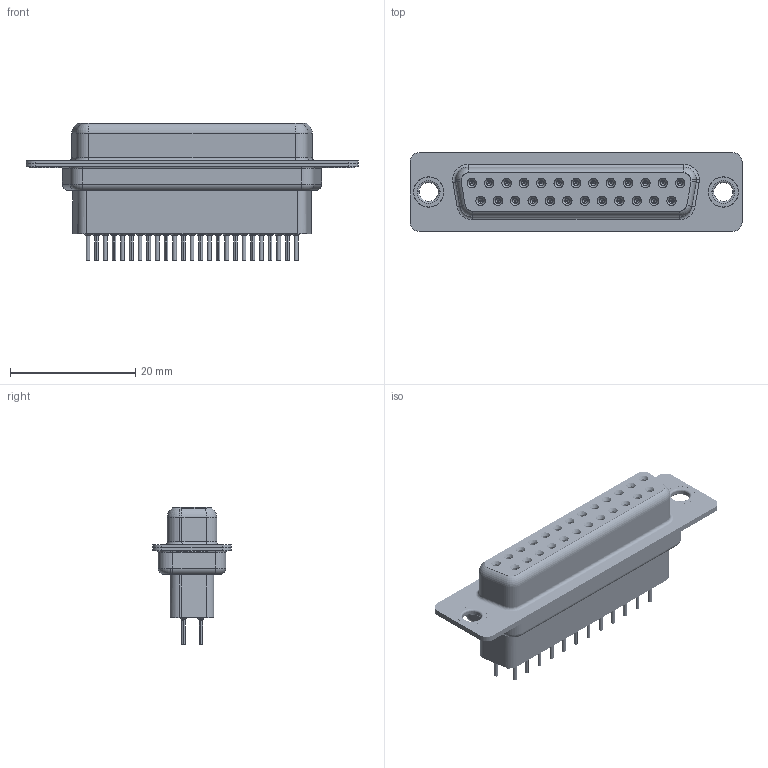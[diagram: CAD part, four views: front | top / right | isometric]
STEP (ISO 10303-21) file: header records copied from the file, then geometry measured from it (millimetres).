
FILE_DESCRIPTION (( 'STEP AP203' ), '1' );
FILE_NAME ('628-025-621-051.STEP', '2020-07-14T15:11:10', ( '' ), ( '' ), 'SwSTEP 2.0', 'SolidWorks 2020', '' );
FILE_SCHEMA (( 'CONFIG_CONTROL_DESIGN' ));
Length unit declared in the file: millimetre
Products named in the file (7): 628 Thru Hole Rivet; 628 Housing_25 HP; 628-025-621-051; 628 Shell Front_25 Contacts; 628 Shell Rear_25 Contacts; 628 Contact Row 1_21H; 628 Contact Row 2_21H
Assembly tree (30 placements, depth 2):
  628-025-621-051
    628 Housing_25 HP
    628 Shell Front_25 Contacts
    628 Shell Rear_25 Contacts
    628 Contact Row 1_21H  x13
    628 Contact Row 2_21H  x12
    628 Thru Hole Rivet  x2
Bounding box: 53 x 12.6 x 21.9 mm (x, y, z)
Volume: 4908.2 mm3; surface area: 11337.4 mm2
Topology: 30 solids, 30 shells, 3328 faces, 8503 edges, 5296 vertices
Faces by surface type: cylinder 946, plane 842, torus 665, bspline 500, cone 375
Entity records: 26075 total; most frequent: CARTESIAN_POINT 6355, DIRECTION 4081, ORIENTED_EDGE 3674, EDGE_CURVE 1837, AXIS2_PLACEMENT_3D 1712, VERTEX_POINT 1155, CIRCLE 941, EDGE_LOOP 926
